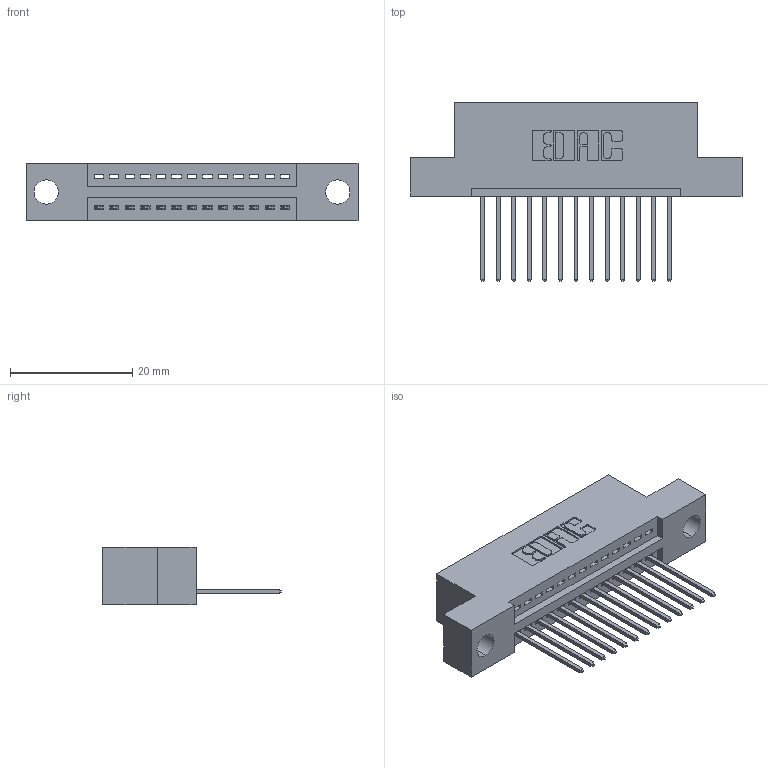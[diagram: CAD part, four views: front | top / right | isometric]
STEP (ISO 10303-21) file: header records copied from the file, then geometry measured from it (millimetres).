
FILE_DESCRIPTION (( 'STEP AP203' ), '1' );
FILE_NAME ('345-013-540-104.STEP', '2021-05-26T14:10:27', ( '' ), ( '' ), 'SwSTEP 2.0', 'SolidWorks 2020', '' );
FILE_SCHEMA (( 'CONFIG_CONTROL_DESIGN' ));
Length unit declared in the file: inch
Products named in the file (3): 345 Part_Flush Mounting Lugs - 0.156 Dia-TI; 345-013-540-104; 345-292-001_345-293-140
Assembly tree (14 placements, depth 2):
  345-013-540-104
    345 Part_Flush Mounting Lugs - 0.156 Dia-TI
    345-292-001_345-293-140  x13
Bounding box: 54.23 x 29.13 x 9.4 mm (x, y, z)
Volume: 4824.8 mm3; surface area: 5986.8 mm2
Topology: 14 solids, 14 shells, 894 faces, 2665 edges, 1758 vertices
Faces by surface type: plane 614, cylinder 280
Entity records: 14125 total; most frequent: CARTESIAN_POINT 2457, ORIENTED_EDGE 2402, DIRECTION 2187, EDGE_CURVE 1201, LINE 1017, VECTOR 1017, VERTEX_POINT 798, AXIS2_PLACEMENT_3D 585
